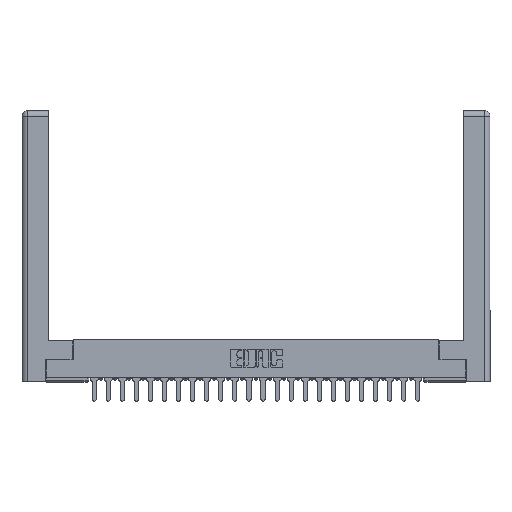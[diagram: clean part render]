
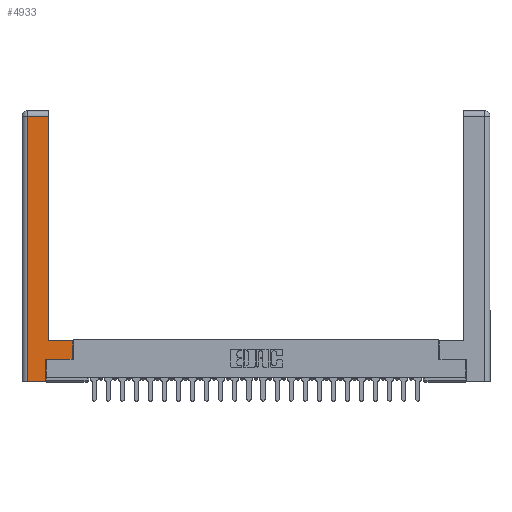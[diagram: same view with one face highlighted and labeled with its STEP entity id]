
A CAD part, top view. The second image highlights one B-rep face of the part: STEP entity #4933.
In plain terms, the highlighted planar face has unit normal (0, 0, 1).
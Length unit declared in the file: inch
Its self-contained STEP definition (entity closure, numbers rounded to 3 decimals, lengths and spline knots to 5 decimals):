
#126 = DIRECTION ( 'NONE',  ( 0., 0., -1. ) ) ;
#783 = LINE ( 'NONE', #10403, #8153 ) ;
#1114 = LINE ( 'NONE', #8343, #6342 ) ;
#1449 = CARTESIAN_POINT ( 'NONE',  ( 0.565, 0.245, 0. ) ) ;
#1884 = DIRECTION ( 'NONE',  ( 0., -1., 0. ) ) ;
#2487 = LINE ( 'NONE', #11649, #14410 ) ;
#3013 = LINE ( 'NONE', #21469, #6698 ) ;
#3032 = DIRECTION ( 'NONE',  ( -1., 0., 0. ) ) ;
#3085 = VERTEX_POINT ( 'NONE', #24601 ) ;
#3314 = CARTESIAN_POINT ( 'NONE',  ( 0., 0., 0. ) ) ;
#3633 = DIRECTION ( 'NONE',  ( 1., 0., 0. ) ) ;
#4933 = ADVANCED_FACE ( 'NONE', ( #5648 ), #8556, .F. ) ;
#5504 = CARTESIAN_POINT ( 'NONE',  ( 0.565, 0.45, 0. ) ) ;
#5648 = FACE_OUTER_BOUND ( 'NONE', #19351, .T. ) ;
#6225 = VERTEX_POINT ( 'NONE', #24994 ) ;
#6342 = VECTOR ( 'NONE', #8604, 39.37008 ) ;
#6698 = VECTOR ( 'NONE', #3633, 39.37008 ) ;
#7321 = EDGE_CURVE ( 'NONE', #10591, #8859, #783, .T. ) ;
#7718 = EDGE_CURVE ( 'NONE', #8859, #6225, #10896, .T. ) ;
#7971 = CARTESIAN_POINT ( 'NONE',  ( 0.265, 0., 0. ) ) ;
#8064 = LINE ( 'NONE', #18807, #16008 ) ;
#8153 = VECTOR ( 'NONE', #20341, 39.37008 ) ;
#8343 = CARTESIAN_POINT ( 'NONE',  ( 0.0615, 2.94, 0. ) ) ;
#8556 = PLANE ( 'NONE',  #24648 ) ;
#8604 = DIRECTION ( 'NONE',  ( -1., 0., 0. ) ) ;
#8859 = VERTEX_POINT ( 'NONE', #17511 ) ;
#9043 = DIRECTION ( 'NONE',  ( -1., 0., 0. ) ) ;
#9333 = VERTEX_POINT ( 'NONE', #10725 ) ;
#9499 = ORIENTED_EDGE ( 'NONE', *, *, #13997, .T. ) ;
#9920 = DIRECTION ( 'NONE',  ( 0., 1., 0. ) ) ;
#10403 = CARTESIAN_POINT ( 'NONE',  ( 0.265, 0.245, 0. ) ) ;
#10524 = EDGE_CURVE ( 'NONE', #20206, #9333, #2487, .T. ) ;
#10591 = VERTEX_POINT ( 'NONE', #7971 ) ;
#10725 = CARTESIAN_POINT ( 'NONE',  ( 0.0615, 0., 0. ) ) ;
#10896 = LINE ( 'NONE', #1449, #13049 ) ;
#11614 = EDGE_CURVE ( 'NONE', #13097, #3085, #8064, .T. ) ;
#11649 = CARTESIAN_POINT ( 'NONE',  ( 0.0615, 0., 0. ) ) ;
#13049 = VECTOR ( 'NONE', #17394, 39.37008 ) ;
#13097 = VERTEX_POINT ( 'NONE', #5504 ) ;
#13850 = CARTESIAN_POINT ( 'NONE',  ( 0.565, 0.45, 0. ) ) ;
#13950 = CARTESIAN_POINT ( 'NONE',  ( 0.295, 2.94, 0. ) ) ;
#13997 = EDGE_CURVE ( 'NONE', #6225, #13097, #24776, .T. ) ;
#14349 = VECTOR ( 'NONE', #9920, 39.37008 ) ;
#14410 = VECTOR ( 'NONE', #1884, 39.37008 ) ;
#14717 = EDGE_CURVE ( 'NONE', #3085, #22822, #17050, .T. ) ;
#14749 = EDGE_CURVE ( 'NONE', #22822, #20206, #1114, .T. ) ;
#15733 = CARTESIAN_POINT ( 'NONE',  ( 0.0615, 2.94, 0. ) ) ;
#15801 = VECTOR ( 'NONE', #18371, 39.37008 ) ;
#16008 = VECTOR ( 'NONE', #9043, 39.37008 ) ;
#17050 = LINE ( 'NONE', #18543, #15801 ) ;
#17394 = DIRECTION ( 'NONE',  ( 1., 0., 0. ) ) ;
#17511 = CARTESIAN_POINT ( 'NONE',  ( 0.265, 0.245, 0. ) ) ;
#18371 = DIRECTION ( 'NONE',  ( 0., 1., 0. ) ) ;
#18543 = CARTESIAN_POINT ( 'NONE',  ( 0.295, 3., 0. ) ) ;
#18807 = CARTESIAN_POINT ( 'NONE',  ( 0.295, 0.45, 0. ) ) ;
#19351 = EDGE_LOOP ( 'NONE', ( #21884, #24724, #20192, #23404, #25081, #22986, #9499, #20388 ) ) ;
#20192 = ORIENTED_EDGE ( 'NONE', *, *, #10524, .T. ) ;
#20206 = VERTEX_POINT ( 'NONE', #15733 ) ;
#20341 = DIRECTION ( 'NONE',  ( 0., 1., 0. ) ) ;
#20388 = ORIENTED_EDGE ( 'NONE', *, *, #11614, .T. ) ;
#21469 = CARTESIAN_POINT ( 'NONE',  ( 0.265, 0., 0. ) ) ;
#21884 = ORIENTED_EDGE ( 'NONE', *, *, #14717, .T. ) ;
#22822 = VERTEX_POINT ( 'NONE', #13950 ) ;
#22986 = ORIENTED_EDGE ( 'NONE', *, *, #7718, .T. ) ;
#23404 = ORIENTED_EDGE ( 'NONE', *, *, #24004, .T. ) ;
#24004 = EDGE_CURVE ( 'NONE', #9333, #10591, #3013, .T. ) ;
#24601 = CARTESIAN_POINT ( 'NONE',  ( 0.295, 0.45, 0. ) ) ;
#24648 = AXIS2_PLACEMENT_3D ( 'NONE', #3314, #126, #3032 ) ;
#24724 = ORIENTED_EDGE ( 'NONE', *, *, #14749, .T. ) ;
#24776 = LINE ( 'NONE', #13850, #14349 ) ;
#24994 = CARTESIAN_POINT ( 'NONE',  ( 0.565, 0.245, 0. ) ) ;
#25081 = ORIENTED_EDGE ( 'NONE', *, *, #7321, .T. ) ;
